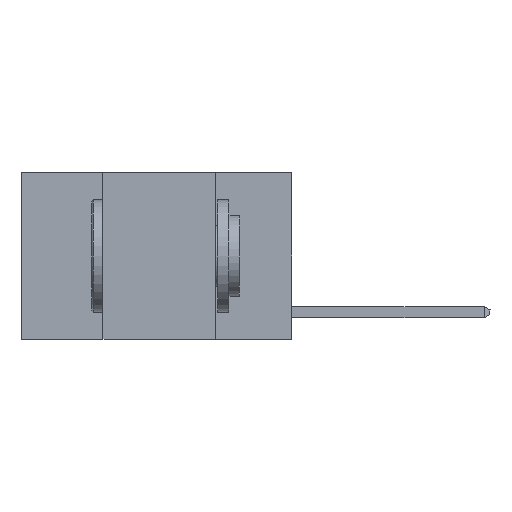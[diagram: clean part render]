
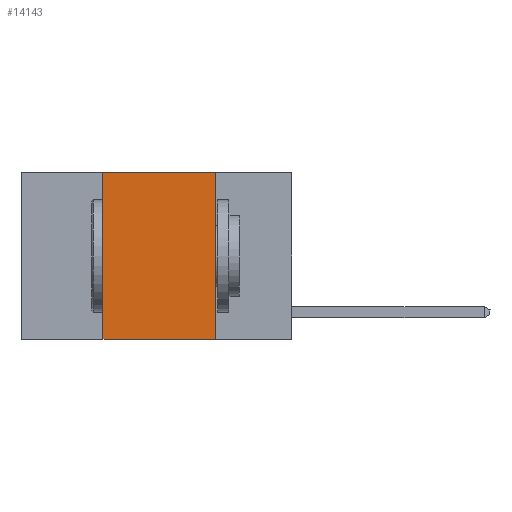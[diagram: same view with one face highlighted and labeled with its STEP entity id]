
A CAD part, left-side view. The second image highlights one B-rep face of the part: STEP entity #14143.
In plain terms, the highlighted planar face has unit normal (-1, 0, 0).
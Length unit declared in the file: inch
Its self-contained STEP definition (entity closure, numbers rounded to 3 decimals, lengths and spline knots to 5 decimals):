
#47 = VECTOR ( 'NONE', #12905, 39.37008 ) ;
#497 = ORIENTED_EDGE ( 'NONE', *, *, #9821, .F. ) ;
#922 = DIRECTION ( 'NONE',  ( 0., -1., 0. ) ) ;
#938 = EDGE_LOOP ( 'NONE', ( #497, #4331, #7657, #14630 ) ) ;
#1934 = VECTOR ( 'NONE', #5931, 39.37008 ) ;
#2569 = CARTESIAN_POINT ( 'NONE',  ( 0., 0.17, -0.37 ) ) ;
#3218 = EDGE_CURVE ( 'NONE', #7570, #6583, #8512, .T. ) ;
#4053 = VERTEX_POINT ( 'NONE', #11834 ) ;
#4331 = ORIENTED_EDGE ( 'NONE', *, *, #3218, .F. ) ;
#4693 = CARTESIAN_POINT ( 'NONE',  ( 0., 0.17, 0. ) ) ;
#5681 = FACE_OUTER_BOUND ( 'NONE', #938, .T. ) ;
#5896 = AXIS2_PLACEMENT_3D ( 'NONE', #14669, #13545, #6045 ) ;
#5931 = DIRECTION ( 'NONE',  ( 0., 0., -1. ) ) ;
#6045 = DIRECTION ( 'NONE',  ( 0., 0., -1. ) ) ;
#6583 = VERTEX_POINT ( 'NONE', #7636 ) ;
#6830 = LINE ( 'NONE', #10302, #47 ) ;
#7329 = CARTESIAN_POINT ( 'NONE',  ( 0., 0.42, 0. ) ) ;
#7570 = VERTEX_POINT ( 'NONE', #15630 ) ;
#7636 = CARTESIAN_POINT ( 'NONE',  ( 0., 0.17, 0. ) ) ;
#7657 = ORIENTED_EDGE ( 'NONE', *, *, #13617, .F. ) ;
#8512 = LINE ( 'NONE', #13258, #11474 ) ;
#9790 = VECTOR ( 'NONE', #9890, 39.37008 ) ;
#9821 = EDGE_CURVE ( 'NONE', #6583, #13769, #11576, .T. ) ;
#9890 = DIRECTION ( 'NONE',  ( 0., 0., 1. ) ) ;
#10196 = LINE ( 'NONE', #7329, #9790 ) ;
#10302 = CARTESIAN_POINT ( 'NONE',  ( 0., 0.6, -0.37 ) ) ;
#11474 = VECTOR ( 'NONE', #922, 39.37008 ) ;
#11576 = LINE ( 'NONE', #4693, #1934 ) ;
#11834 = CARTESIAN_POINT ( 'NONE',  ( 0., 0.42, -0.37 ) ) ;
#12905 = DIRECTION ( 'NONE',  ( 0., -1., 0. ) ) ;
#13258 = CARTESIAN_POINT ( 'NONE',  ( 0., 0.6, 0. ) ) ;
#13431 = PLANE ( 'NONE',  #5896 ) ;
#13545 = DIRECTION ( 'NONE',  ( 1., 0., 0. ) ) ;
#13617 = EDGE_CURVE ( 'NONE', #4053, #7570, #10196, .T. ) ;
#13769 = VERTEX_POINT ( 'NONE', #2569 ) ;
#14143 = ADVANCED_FACE ( 'NONE', ( #5681 ), #13431, .F. ) ;
#14483 = EDGE_CURVE ( 'NONE', #4053, #13769, #6830, .T. ) ;
#14630 = ORIENTED_EDGE ( 'NONE', *, *, #14483, .T. ) ;
#14669 = CARTESIAN_POINT ( 'NONE',  ( 0., 0.6, 0. ) ) ;
#15630 = CARTESIAN_POINT ( 'NONE',  ( 0., 0.42, 0. ) ) ;
